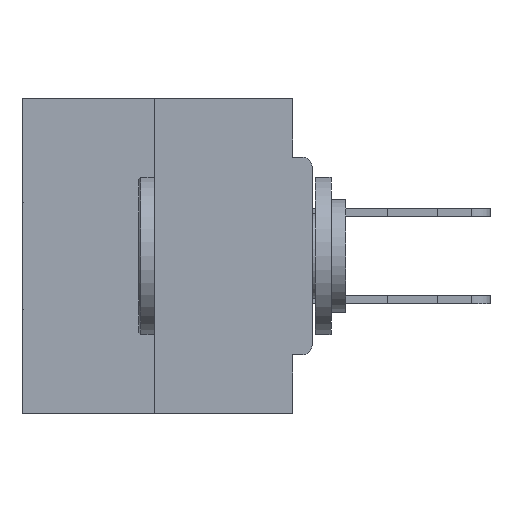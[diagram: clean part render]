
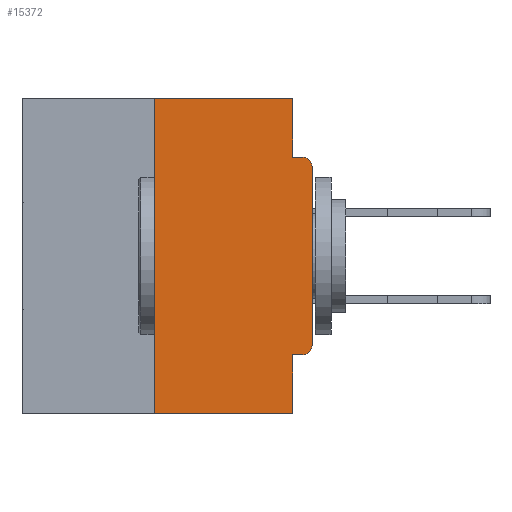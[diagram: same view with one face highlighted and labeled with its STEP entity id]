
A CAD part, left-side view. The second image highlights one B-rep face of the part: STEP entity #15372.
In plain terms, the highlighted planar face has unit normal (-1, 0, 0).
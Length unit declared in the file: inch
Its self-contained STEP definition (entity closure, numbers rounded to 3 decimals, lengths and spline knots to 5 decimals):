
#694 = DIRECTION ( 'NONE',  ( 1., 0., 0. ) ) ;
#826 = DIRECTION ( 'NONE',  ( 0., 0., -1. ) ) ;
#858 = EDGE_CURVE ( 'NONE', #13928, #14039, #15161, .T. ) ;
#1376 = ORIENTED_EDGE ( 'NONE', *, *, #20472, .T. ) ;
#1435 = ORIENTED_EDGE ( 'NONE', *, *, #25496, .F. ) ;
#1482 = DIRECTION ( 'NONE',  ( 0., 0., 1. ) ) ;
#1489 = LINE ( 'NONE', #12851, #33216 ) ;
#1506 = DIRECTION ( 'NONE',  ( 0., 1., 0. ) ) ;
#1579 = ORIENTED_EDGE ( 'NONE', *, *, #7344, .F. ) ;
#1607 = ORIENTED_EDGE ( 'NONE', *, *, #32286, .T. ) ;
#2211 = EDGE_LOOP ( 'NONE', ( #1579, #6775, #1376, #1435, #38453, #7433, #1607, #18322, #28359, #19324 ) ) ;
#4180 = PLANE ( 'NONE',  #4667 ) ;
#4311 = CARTESIAN_POINT ( 'NONE',  ( 0., 0.031, -0.0935 ) ) ;
#4667 = AXIS2_PLACEMENT_3D ( 'NONE', #19282, #694, #826 ) ;
#4746 = EDGE_CURVE ( 'NONE', #7713, #36382, #30400, .T. ) ;
#4977 = VERTEX_POINT ( 'NONE', #28185 ) ;
#6775 = ORIENTED_EDGE ( 'NONE', *, *, #39737, .F. ) ;
#7121 = DIRECTION ( 'NONE',  ( 0., 0., -1. ) ) ;
#7344 = EDGE_CURVE ( 'NONE', #17165, #29076, #1489, .T. ) ;
#7433 = ORIENTED_EDGE ( 'NONE', *, *, #4746, .T. ) ;
#7713 = VERTEX_POINT ( 'NONE', #26786 ) ;
#8092 = CARTESIAN_POINT ( 'NONE',  ( 0., 0.015, -0.3915 ) ) ;
#8129 = DIRECTION ( 'NONE',  ( 0., 0., 1. ) ) ;
#9883 = EDGE_CURVE ( 'NONE', #7713, #4977, #26115, .T. ) ;
#10267 = CARTESIAN_POINT ( 'NONE',  ( 0., 0.015, -0.0935 ) ) ;
#11059 = DIRECTION ( 'NONE',  ( 0., 0., -1. ) ) ;
#12298 = DIRECTION ( 'NONE',  ( 0., -1., 0. ) ) ;
#12851 = CARTESIAN_POINT ( 'NONE',  ( 0., 0.46, 0. ) ) ;
#12943 = CARTESIAN_POINT ( 'NONE',  ( 0., 0.015, -0.1085 ) ) ;
#12979 = DIRECTION ( 'NONE',  ( 0., -1., 0. ) ) ;
#13928 = VERTEX_POINT ( 'NONE', #4311 ) ;
#14039 = VERTEX_POINT ( 'NONE', #10267 ) ;
#14125 = VECTOR ( 'NONE', #1506, 39.37008 ) ;
#14397 = CARTESIAN_POINT ( 'NONE',  ( 0., 0.46, -0.5 ) ) ;
#15161 = LINE ( 'NONE', #24413, #36741 ) ;
#15372 = ADVANCED_FACE ( 'NONE', ( #26135 ), #4180, .F. ) ;
#15399 = EDGE_CURVE ( 'NONE', #23051, #14039, #27087, .T. ) ;
#17165 = VERTEX_POINT ( 'NONE', #36128 ) ;
#17394 = CARTESIAN_POINT ( 'NONE',  ( 0., 0., -0.1085 ) ) ;
#18322 = ORIENTED_EDGE ( 'NONE', *, *, #15399, .T. ) ;
#18746 = EDGE_CURVE ( 'NONE', #29076, #13928, #27472, .T. ) ;
#19282 = CARTESIAN_POINT ( 'NONE',  ( 0., 0.46, 0. ) ) ;
#19324 = ORIENTED_EDGE ( 'NONE', *, *, #18746, .F. ) ;
#20472 = EDGE_CURVE ( 'NONE', #30556, #32908, #39146, .T. ) ;
#22517 = DIRECTION ( 'NONE',  ( 0., 0., -1. ) ) ;
#22830 = VECTOR ( 'NONE', #26735, 39.37008 ) ;
#23051 = VERTEX_POINT ( 'NONE', #17394 ) ;
#23296 = LINE ( 'NONE', #33114, #29061 ) ;
#23848 = CARTESIAN_POINT ( 'NONE',  ( 0., 0.031, -0.5 ) ) ;
#24413 = CARTESIAN_POINT ( 'NONE',  ( 0., 0., -0.0935 ) ) ;
#24657 = CARTESIAN_POINT ( 'NONE',  ( 0., 0.031, -0.5 ) ) ;
#25496 = EDGE_CURVE ( 'NONE', #4977, #32908, #26498, .T. ) ;
#26006 = CARTESIAN_POINT ( 'NONE',  ( 0., 0., -0.4065 ) ) ;
#26115 = LINE ( 'NONE', #26006, #14125 ) ;
#26135 = FACE_OUTER_BOUND ( 'NONE', #2211, .T. ) ;
#26391 = DIRECTION ( 'NONE',  ( -1., 0., 0. ) ) ;
#26498 = LINE ( 'NONE', #23848, #31738 ) ;
#26735 = DIRECTION ( 'NONE',  ( 0., -1., 0. ) ) ;
#26786 = CARTESIAN_POINT ( 'NONE',  ( 0., 0.015, -0.4065 ) ) ;
#27087 = CIRCLE ( 'NONE', #28885, 0.015 ) ;
#27472 = LINE ( 'NONE', #28098, #28933 ) ;
#28098 = CARTESIAN_POINT ( 'NONE',  ( 0., 0.031, 0. ) ) ;
#28185 = CARTESIAN_POINT ( 'NONE',  ( 0., 0.031, -0.4065 ) ) ;
#28359 = ORIENTED_EDGE ( 'NONE', *, *, #858, .F. ) ;
#28885 = AXIS2_PLACEMENT_3D ( 'NONE', #12943, #34397, #22517 ) ;
#28933 = VECTOR ( 'NONE', #7121, 39.37008 ) ;
#29061 = VECTOR ( 'NONE', #8129, 39.37008 ) ;
#29076 = VERTEX_POINT ( 'NONE', #38735 ) ;
#29389 = CARTESIAN_POINT ( 'NONE',  ( 0., 0., -0.3915 ) ) ;
#30098 = CARTESIAN_POINT ( 'NONE',  ( 0., 0.25, -0.5 ) ) ;
#30280 = DIRECTION ( 'NONE',  ( 0., 0., -1. ) ) ;
#30400 = CIRCLE ( 'NONE', #34490, 0.015 ) ;
#30556 = VERTEX_POINT ( 'NONE', #30098 ) ;
#31738 = VECTOR ( 'NONE', #30280, 39.37008 ) ;
#32286 = EDGE_CURVE ( 'NONE', #36382, #23051, #23296, .T. ) ;
#32908 = VERTEX_POINT ( 'NONE', #24657 ) ;
#33114 = CARTESIAN_POINT ( 'NONE',  ( 0., 0., 0. ) ) ;
#33216 = VECTOR ( 'NONE', #12979, 39.37008 ) ;
#34397 = DIRECTION ( 'NONE',  ( -1., 0., 0. ) ) ;
#34490 = AXIS2_PLACEMENT_3D ( 'NONE', #8092, #26391, #11059 ) ;
#35537 = LINE ( 'NONE', #35734, #36970 ) ;
#35734 = CARTESIAN_POINT ( 'NONE',  ( 0., 0.25, 0. ) ) ;
#36128 = CARTESIAN_POINT ( 'NONE',  ( 0., 0.25, 0. ) ) ;
#36382 = VERTEX_POINT ( 'NONE', #29389 ) ;
#36741 = VECTOR ( 'NONE', #12298, 39.37008 ) ;
#36970 = VECTOR ( 'NONE', #1482, 39.37008 ) ;
#38453 = ORIENTED_EDGE ( 'NONE', *, *, #9883, .F. ) ;
#38735 = CARTESIAN_POINT ( 'NONE',  ( 0., 0.031, 0. ) ) ;
#39146 = LINE ( 'NONE', #14397, #22830 ) ;
#39737 = EDGE_CURVE ( 'NONE', #30556, #17165, #35537, .T. ) ;
